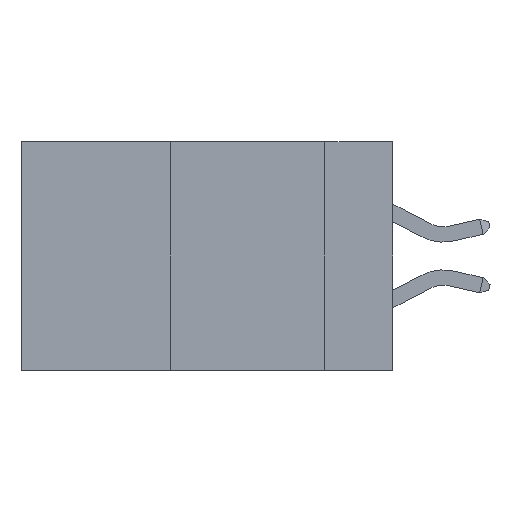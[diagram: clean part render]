
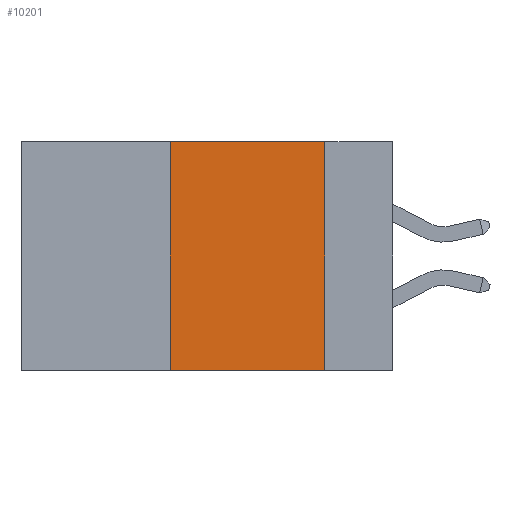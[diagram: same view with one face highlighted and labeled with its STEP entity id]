
A CAD part, left-side view. The second image highlights one B-rep face of the part: STEP entity #10201.
In plain terms, the highlighted planar face has unit normal (-1, 0, 0).
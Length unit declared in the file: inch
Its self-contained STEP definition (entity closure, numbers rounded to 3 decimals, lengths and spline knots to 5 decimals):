
#2995 = EDGE_CURVE ( 'NONE', #23344, #29406, #28278, .T. ) ;
#5565 = CARTESIAN_POINT ( 'NONE',  ( 0., 0.36, -0.37 ) ) ;
#6301 = EDGE_CURVE ( 'NONE', #13341, #23344, #28069, .T. ) ;
#8067 = DIRECTION ( 'NONE',  ( 0., 0., 1. ) ) ;
#8545 = DIRECTION ( 'NONE',  ( 0., -1., 0. ) ) ;
#9781 = LINE ( 'NONE', #17977, #19747 ) ;
#9858 = PLANE ( 'NONE',  #27793 ) ;
#10201 = ADVANCED_FACE ( 'NONE', ( #16149 ), #9858, .F. ) ;
#10314 = CARTESIAN_POINT ( 'NONE',  ( 0., 0.36, 0. ) ) ;
#10975 = CARTESIAN_POINT ( 'NONE',  ( 0., 0.11, 0. ) ) ;
#11351 = CARTESIAN_POINT ( 'NONE',  ( 0., 0.11, -0.37 ) ) ;
#12139 = DIRECTION ( 'NONE',  ( 1., 0., 0. ) ) ;
#13341 = VERTEX_POINT ( 'NONE', #14995 ) ;
#14995 = CARTESIAN_POINT ( 'NONE',  ( 0., 0.36, 0. ) ) ;
#15895 = VECTOR ( 'NONE', #8067, 39.37008 ) ;
#16149 = FACE_OUTER_BOUND ( 'NONE', #19954, .T. ) ;
#16159 = VECTOR ( 'NONE', #24344, 39.37008 ) ;
#17292 = CARTESIAN_POINT ( 'NONE',  ( 0., 0.6, 0. ) ) ;
#17977 = CARTESIAN_POINT ( 'NONE',  ( 0., 0.6, -0.37 ) ) ;
#18342 = CARTESIAN_POINT ( 'NONE',  ( 0., 0.11, 0. ) ) ;
#18615 = DIRECTION ( 'NONE',  ( 0., 0., -1. ) ) ;
#19747 = VECTOR ( 'NONE', #20288, 39.37008 ) ;
#19954 = EDGE_LOOP ( 'NONE', ( #24145, #21919, #22326, #24406 ) ) ;
#20288 = DIRECTION ( 'NONE',  ( 0., -1., 0. ) ) ;
#20526 = EDGE_CURVE ( 'NONE', #20979, #29406, #9781, .T. ) ;
#20979 = VERTEX_POINT ( 'NONE', #5565 ) ;
#21919 = ORIENTED_EDGE ( 'NONE', *, *, #6301, .F. ) ;
#21979 = LINE ( 'NONE', #10314, #15895 ) ;
#22326 = ORIENTED_EDGE ( 'NONE', *, *, #25201, .F. ) ;
#23344 = VERTEX_POINT ( 'NONE', #18342 ) ;
#24145 = ORIENTED_EDGE ( 'NONE', *, *, #2995, .F. ) ;
#24344 = DIRECTION ( 'NONE',  ( 0., 0., -1. ) ) ;
#24406 = ORIENTED_EDGE ( 'NONE', *, *, #20526, .T. ) ;
#24937 = VECTOR ( 'NONE', #8545, 39.37008 ) ;
#25201 = EDGE_CURVE ( 'NONE', #20979, #13341, #21979, .T. ) ;
#25799 = CARTESIAN_POINT ( 'NONE',  ( 0., 0.6, 0. ) ) ;
#27793 = AXIS2_PLACEMENT_3D ( 'NONE', #25799, #12139, #18615 ) ;
#28069 = LINE ( 'NONE', #17292, #24937 ) ;
#28278 = LINE ( 'NONE', #10975, #16159 ) ;
#29406 = VERTEX_POINT ( 'NONE', #11351 ) ;
